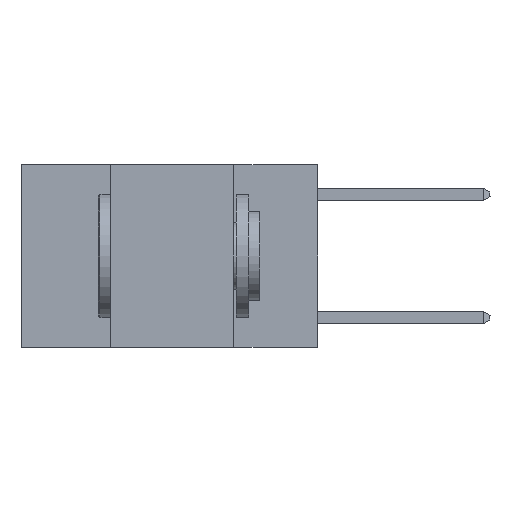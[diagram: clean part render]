
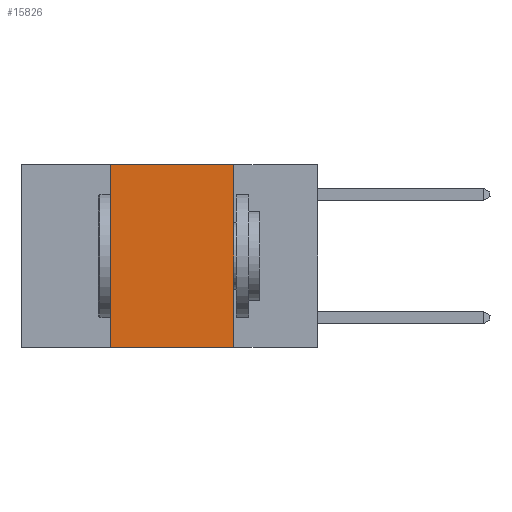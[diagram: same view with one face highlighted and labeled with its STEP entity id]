
A CAD part, left-side view. The second image highlights one B-rep face of the part: STEP entity #15826.
In plain terms, the highlighted planar face has unit normal (-1, 0, 0).
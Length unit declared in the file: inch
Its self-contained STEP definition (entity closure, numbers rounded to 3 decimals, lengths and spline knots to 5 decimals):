
#632 = LINE ( 'NONE', #4943, #18781 ) ;
#713 = LINE ( 'NONE', #8813, #1801 ) ;
#888 = CARTESIAN_POINT ( 'NONE',  ( 0., 0.6, 0. ) ) ;
#1140 = CARTESIAN_POINT ( 'NONE',  ( 0., 0.42, 0. ) ) ;
#1263 = DIRECTION ( 'NONE',  ( 0., -1., 0. ) ) ;
#1801 = VECTOR ( 'NONE', #8679, 39.37008 ) ;
#4064 = VERTEX_POINT ( 'NONE', #11971 ) ;
#4943 = CARTESIAN_POINT ( 'NONE',  ( 0., 0.42, 0. ) ) ;
#5551 = EDGE_LOOP ( 'NONE', ( #21489, #18311, #5637, #22385 ) ) ;
#5637 = ORIENTED_EDGE ( 'NONE', *, *, #20577, .F. ) ;
#6935 = CARTESIAN_POINT ( 'NONE',  ( 0., 0.42, -0.37 ) ) ;
#8679 = DIRECTION ( 'NONE',  ( 0., 0., -1. ) ) ;
#8813 = CARTESIAN_POINT ( 'NONE',  ( 0., 0.17, 0. ) ) ;
#9353 = DIRECTION ( 'NONE',  ( 1., 0., 0. ) ) ;
#10988 = DIRECTION ( 'NONE',  ( 0., 0., -1. ) ) ;
#11971 = CARTESIAN_POINT ( 'NONE',  ( 0., 0.17, 0. ) ) ;
#12543 = LINE ( 'NONE', #888, #19508 ) ;
#14718 = VECTOR ( 'NONE', #1263, 39.37008 ) ;
#15065 = PLANE ( 'NONE',  #19486 ) ;
#15435 = CARTESIAN_POINT ( 'NONE',  ( 0., 0.6, 0. ) ) ;
#15647 = EDGE_CURVE ( 'NONE', #21884, #4064, #12543, .T. ) ;
#15826 = ADVANCED_FACE ( 'NONE', ( #24822 ), #15065, .F. ) ;
#16706 = LINE ( 'NONE', #18690, #14718 ) ;
#16954 = EDGE_CURVE ( 'NONE', #17416, #18130, #16706, .T. ) ;
#17416 = VERTEX_POINT ( 'NONE', #6935 ) ;
#17876 = EDGE_CURVE ( 'NONE', #4064, #18130, #713, .T. ) ;
#18130 = VERTEX_POINT ( 'NONE', #21420 ) ;
#18311 = ORIENTED_EDGE ( 'NONE', *, *, #15647, .F. ) ;
#18690 = CARTESIAN_POINT ( 'NONE',  ( 0., 0.6, -0.37 ) ) ;
#18781 = VECTOR ( 'NONE', #19971, 39.37008 ) ;
#19486 = AXIS2_PLACEMENT_3D ( 'NONE', #15435, #9353, #10988 ) ;
#19508 = VECTOR ( 'NONE', #24452, 39.37008 ) ;
#19971 = DIRECTION ( 'NONE',  ( 0., 0., 1. ) ) ;
#20577 = EDGE_CURVE ( 'NONE', #17416, #21884, #632, .T. ) ;
#21420 = CARTESIAN_POINT ( 'NONE',  ( 0., 0.17, -0.37 ) ) ;
#21489 = ORIENTED_EDGE ( 'NONE', *, *, #17876, .F. ) ;
#21884 = VERTEX_POINT ( 'NONE', #1140 ) ;
#22385 = ORIENTED_EDGE ( 'NONE', *, *, #16954, .T. ) ;
#24452 = DIRECTION ( 'NONE',  ( 0., -1., 0. ) ) ;
#24822 = FACE_OUTER_BOUND ( 'NONE', #5551, .T. ) ;
